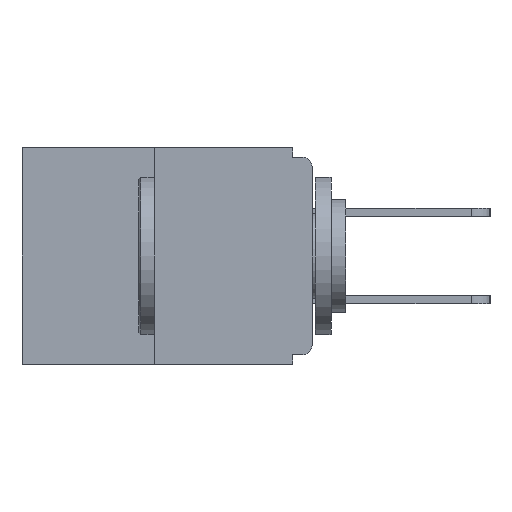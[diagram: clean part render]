
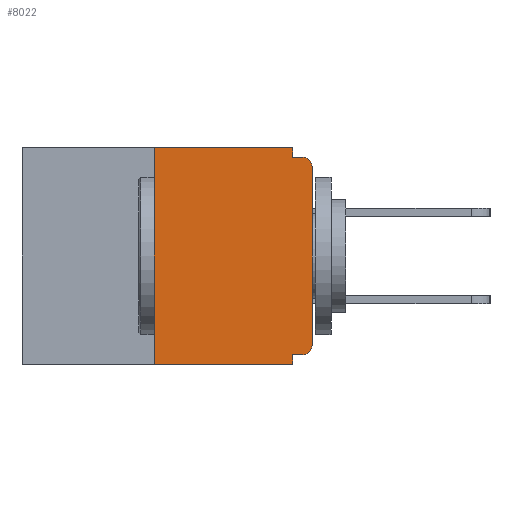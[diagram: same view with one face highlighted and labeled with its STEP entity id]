
A CAD part, left-side view. The second image highlights one B-rep face of the part: STEP entity #8022.
In plain terms, the highlighted planar face has unit normal (-1, 0, 0).
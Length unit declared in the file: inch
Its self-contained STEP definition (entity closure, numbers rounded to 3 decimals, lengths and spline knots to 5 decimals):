
#108 = VECTOR ( 'NONE', #10664, 39.37008 ) ;
#233 = ORIENTED_EDGE ( 'NONE', *, *, #7659, .T. ) ;
#338 = ORIENTED_EDGE ( 'NONE', *, *, #4854, .T. ) ;
#427 = EDGE_CURVE ( 'NONE', #4436, #4822, #14617, .T. ) ;
#509 = DIRECTION ( 'NONE',  ( 0., 1., 0. ) ) ;
#779 = VECTOR ( 'NONE', #5772, 39.37008 ) ;
#785 = VECTOR ( 'NONE', #14299, 39.37008 ) ;
#829 = ORIENTED_EDGE ( 'NONE', *, *, #427, .T. ) ;
#978 = DIRECTION ( 'NONE',  ( 0., -1., 0. ) ) ;
#1053 = DIRECTION ( 'NONE',  ( -1., 0., 0. ) ) ;
#1287 = VECTOR ( 'NONE', #509, 39.37008 ) ;
#1530 = CARTESIAN_POINT ( 'NONE',  ( 0., 0., -0.015 ) ) ;
#2682 = VERTEX_POINT ( 'NONE', #16385 ) ;
#2752 = CARTESIAN_POINT ( 'NONE',  ( 0., 0.031, 0. ) ) ;
#2761 = CIRCLE ( 'NONE', #18593, 0.015 ) ;
#2778 = ORIENTED_EDGE ( 'NONE', *, *, #17570, .T. ) ;
#3017 = LINE ( 'NONE', #12119, #108 ) ;
#3270 = CARTESIAN_POINT ( 'NONE',  ( 0., 0., -0.328 ) ) ;
#3771 = CARTESIAN_POINT ( 'NONE',  ( 0., 0.015, -0.03 ) ) ;
#3904 = VECTOR ( 'NONE', #11717, 39.37008 ) ;
#3936 = CARTESIAN_POINT ( 'NONE',  ( 0., 0.46, -0.343 ) ) ;
#3965 = CARTESIAN_POINT ( 'NONE',  ( 0., 0.25, 0. ) ) ;
#4436 = VERTEX_POINT ( 'NONE', #18150 ) ;
#4822 = VERTEX_POINT ( 'NONE', #15306 ) ;
#4854 = EDGE_CURVE ( 'NONE', #17961, #15089, #12569, .T. ) ;
#5161 = LINE ( 'NONE', #2752, #13743 ) ;
#5242 = DIRECTION ( 'NONE',  ( -1., 0., 0. ) ) ;
#5517 = CARTESIAN_POINT ( 'NONE',  ( 0., 0.015, -0.015 ) ) ;
#5772 = DIRECTION ( 'NONE',  ( 0., -1., 0. ) ) ;
#5775 = CARTESIAN_POINT ( 'NONE',  ( 0., 0.25, 0. ) ) ;
#6346 = AXIS2_PLACEMENT_3D ( 'NONE', #11034, #15331, #15453 ) ;
#6562 = EDGE_CURVE ( 'NONE', #17558, #2682, #11162, .T. ) ;
#6654 = ORIENTED_EDGE ( 'NONE', *, *, #15598, .F. ) ;
#6662 = VERTEX_POINT ( 'NONE', #17610 ) ;
#7052 = LINE ( 'NONE', #13104, #3904 ) ;
#7659 = EDGE_CURVE ( 'NONE', #15089, #11983, #3017, .T. ) ;
#7718 = EDGE_LOOP ( 'NONE', ( #16491, #6654, #829, #13856, #8894, #338, #233, #2778, #18305, #15951 ) ) ;
#8022 = ADVANCED_FACE ( 'NONE', ( #12070 ), #14318, .F. ) ;
#8289 = VECTOR ( 'NONE', #978, 39.37008 ) ;
#8811 = DIRECTION ( 'NONE',  ( 0., 0., -1. ) ) ;
#8894 = ORIENTED_EDGE ( 'NONE', *, *, #15243, .F. ) ;
#10523 = VECTOR ( 'NONE', #16033, 39.37008 ) ;
#10664 = DIRECTION ( 'NONE',  ( 0., 0., 1. ) ) ;
#11034 = CARTESIAN_POINT ( 'NONE',  ( 0., 0.46, 0. ) ) ;
#11162 = LINE ( 'NONE', #14418, #779 ) ;
#11717 = DIRECTION ( 'NONE',  ( 0., 0., -1. ) ) ;
#11983 = VERTEX_POINT ( 'NONE', #15564 ) ;
#12070 = FACE_OUTER_BOUND ( 'NONE', #7718, .T. ) ;
#12119 = CARTESIAN_POINT ( 'NONE',  ( 0., 0., 0. ) ) ;
#12282 = CARTESIAN_POINT ( 'NONE',  ( 0., 0.031, -0.015 ) ) ;
#12474 = CARTESIAN_POINT ( 'NONE',  ( 0., 0.015, -0.313 ) ) ;
#12569 = CIRCLE ( 'NONE', #13529, 0.015 ) ;
#12800 = LINE ( 'NONE', #3270, #1287 ) ;
#13104 = CARTESIAN_POINT ( 'NONE',  ( 0., 0.031, -0.343 ) ) ;
#13529 = AXIS2_PLACEMENT_3D ( 'NONE', #12474, #1053, #15371 ) ;
#13743 = VECTOR ( 'NONE', #8811, 39.37008 ) ;
#13856 = ORIENTED_EDGE ( 'NONE', *, *, #17851, .F. ) ;
#14076 = EDGE_CURVE ( 'NONE', #2682, #16086, #5161, .T. ) ;
#14299 = DIRECTION ( 'NONE',  ( 0., 0., 1. ) ) ;
#14318 = PLANE ( 'NONE',  #6346 ) ;
#14418 = CARTESIAN_POINT ( 'NONE',  ( 0., 0.46, 0. ) ) ;
#14617 = LINE ( 'NONE', #3936, #8289 ) ;
#14900 = VERTEX_POINT ( 'NONE', #5517 ) ;
#14985 = CARTESIAN_POINT ( 'NONE',  ( 0., 0.015, -0.328 ) ) ;
#15089 = VERTEX_POINT ( 'NONE', #17667 ) ;
#15126 = EDGE_CURVE ( 'NONE', #16086, #14900, #16625, .T. ) ;
#15243 = EDGE_CURVE ( 'NONE', #17961, #6662, #12800, .T. ) ;
#15306 = CARTESIAN_POINT ( 'NONE',  ( 0., 0.031, -0.343 ) ) ;
#15331 = DIRECTION ( 'NONE',  ( 1., 0., 0. ) ) ;
#15337 = DIRECTION ( 'NONE',  ( 0., 0., -1. ) ) ;
#15371 = DIRECTION ( 'NONE',  ( 0., 0., -1. ) ) ;
#15453 = DIRECTION ( 'NONE',  ( 0., 0., -1. ) ) ;
#15564 = CARTESIAN_POINT ( 'NONE',  ( 0., 0., -0.03 ) ) ;
#15598 = EDGE_CURVE ( 'NONE', #4436, #17558, #16589, .T. ) ;
#15951 = ORIENTED_EDGE ( 'NONE', *, *, #14076, .F. ) ;
#16033 = DIRECTION ( 'NONE',  ( 0., -1., 0. ) ) ;
#16086 = VERTEX_POINT ( 'NONE', #12282 ) ;
#16385 = CARTESIAN_POINT ( 'NONE',  ( 0., 0.031, 0. ) ) ;
#16491 = ORIENTED_EDGE ( 'NONE', *, *, #6562, .F. ) ;
#16589 = LINE ( 'NONE', #5775, #785 ) ;
#16625 = LINE ( 'NONE', #1530, #10523 ) ;
#17558 = VERTEX_POINT ( 'NONE', #3965 ) ;
#17570 = EDGE_CURVE ( 'NONE', #11983, #14900, #2761, .T. ) ;
#17610 = CARTESIAN_POINT ( 'NONE',  ( 0., 0.031, -0.328 ) ) ;
#17667 = CARTESIAN_POINT ( 'NONE',  ( 0., 0., -0.313 ) ) ;
#17851 = EDGE_CURVE ( 'NONE', #6662, #4822, #7052, .T. ) ;
#17961 = VERTEX_POINT ( 'NONE', #14985 ) ;
#18150 = CARTESIAN_POINT ( 'NONE',  ( 0., 0.25, -0.343 ) ) ;
#18305 = ORIENTED_EDGE ( 'NONE', *, *, #15126, .F. ) ;
#18593 = AXIS2_PLACEMENT_3D ( 'NONE', #3771, #5242, #15337 ) ;
